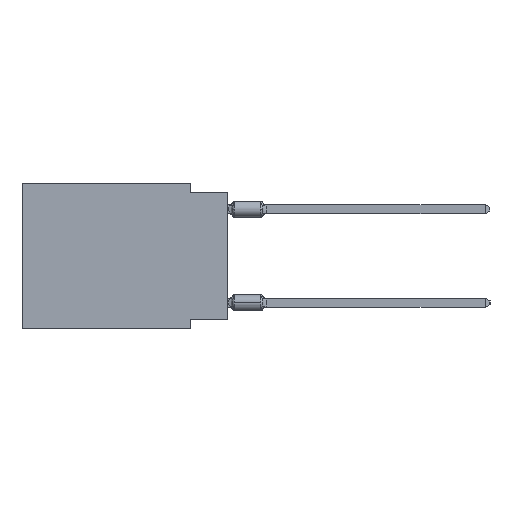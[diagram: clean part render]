
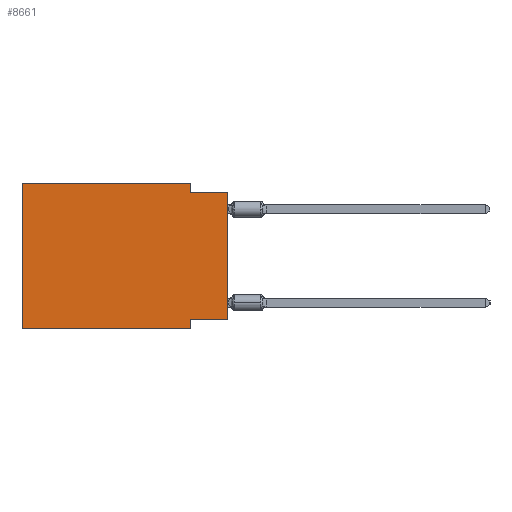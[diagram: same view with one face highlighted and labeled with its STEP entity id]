
A CAD part, left-side view. The second image highlights one B-rep face of the part: STEP entity #8661.
In plain terms, the highlighted planar face has unit normal (-1, 0, 0).
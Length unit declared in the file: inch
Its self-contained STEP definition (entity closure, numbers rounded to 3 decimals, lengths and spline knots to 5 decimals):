
#216 = CARTESIAN_POINT ( 'NONE',  ( 0., 0.1, -0.025 ) ) ;
#1521 = LINE ( 'NONE', #36367, #37844 ) ;
#1956 = ORIENTED_EDGE ( 'NONE', *, *, #28556, .F. ) ;
#2195 = CARTESIAN_POINT ( 'NONE',  ( 0., 0.1, 0. ) ) ;
#2839 = CARTESIAN_POINT ( 'NONE',  ( 0., 0.55, -0.39 ) ) ;
#4814 = LINE ( 'NONE', #23485, #38915 ) ;
#5425 = ORIENTED_EDGE ( 'NONE', *, *, #21490, .F. ) ;
#6575 = EDGE_CURVE ( 'NONE', #15605, #26968, #23163, .T. ) ;
#7314 = VERTEX_POINT ( 'NONE', #25768 ) ;
#8661 = ADVANCED_FACE ( 'NONE', ( #19843 ), #29776, .F. ) ;
#9729 = ORIENTED_EDGE ( 'NONE', *, *, #18205, .F. ) ;
#10688 = DIRECTION ( 'NONE',  ( 1., 0., 0. ) ) ;
#10963 = DIRECTION ( 'NONE',  ( 0., 0., 1. ) ) ;
#11843 = DIRECTION ( 'NONE',  ( 0., -1., 0. ) ) ;
#12040 = CARTESIAN_POINT ( 'NONE',  ( 0., 0.55, 0. ) ) ;
#12055 = CARTESIAN_POINT ( 'NONE',  ( 0., 0.1, -0.39 ) ) ;
#12072 = VERTEX_POINT ( 'NONE', #216 ) ;
#12468 = DIRECTION ( 'NONE',  ( 0., 0., 1. ) ) ;
#13388 = ORIENTED_EDGE ( 'NONE', *, *, #16372, .T. ) ;
#13749 = DIRECTION ( 'NONE',  ( 0., 1., 0. ) ) ;
#14763 = VECTOR ( 'NONE', #12468, 39.37008 ) ;
#15605 = VERTEX_POINT ( 'NONE', #2839 ) ;
#16372 = EDGE_CURVE ( 'NONE', #22951, #7314, #34476, .T. ) ;
#16384 = DIRECTION ( 'NONE',  ( 0., 0., -1. ) ) ;
#17668 = LINE ( 'NONE', #12040, #34386 ) ;
#17761 = DIRECTION ( 'NONE',  ( 0., 0., -1. ) ) ;
#18205 = EDGE_CURVE ( 'NONE', #35127, #26968, #38156, .T. ) ;
#19767 = VECTOR ( 'NONE', #17761, 39.37008 ) ;
#19843 = FACE_OUTER_BOUND ( 'NONE', #28396, .T. ) ;
#19909 = CARTESIAN_POINT ( 'NONE',  ( 0., 0.1, -0.39 ) ) ;
#20731 = ORIENTED_EDGE ( 'NONE', *, *, #25065, .F. ) ;
#21490 = EDGE_CURVE ( 'NONE', #22951, #35127, #4814, .T. ) ;
#21963 = CARTESIAN_POINT ( 'NONE',  ( 0., 0., -0.365 ) ) ;
#22441 = CARTESIAN_POINT ( 'NONE',  ( 0., 0.55, 0. ) ) ;
#22951 = VERTEX_POINT ( 'NONE', #21963 ) ;
#23114 = EDGE_CURVE ( 'NONE', #15605, #38725, #27157, .T. ) ;
#23163 = LINE ( 'NONE', #36211, #34443 ) ;
#23334 = DIRECTION ( 'NONE',  ( 0., 0., -1. ) ) ;
#23485 = CARTESIAN_POINT ( 'NONE',  ( 0., 0., -0.365 ) ) ;
#23658 = VECTOR ( 'NONE', #10963, 39.37008 ) ;
#24679 = CARTESIAN_POINT ( 'NONE',  ( 0., 0.1, 0. ) ) ;
#25065 = EDGE_CURVE ( 'NONE', #38725, #37426, #17668, .T. ) ;
#25768 = CARTESIAN_POINT ( 'NONE',  ( 0., 0., -0.025 ) ) ;
#26687 = LINE ( 'NONE', #2195, #19767 ) ;
#26968 = VERTEX_POINT ( 'NONE', #12055 ) ;
#27035 = DIRECTION ( 'NONE',  ( 0., -1., 0. ) ) ;
#27157 = LINE ( 'NONE', #39802, #23658 ) ;
#28396 = EDGE_LOOP ( 'NONE', ( #13388, #1956, #31101, #20731, #38252, #34993, #9729, #5425 ) ) ;
#28556 = EDGE_CURVE ( 'NONE', #12072, #7314, #1521, .T. ) ;
#29776 = PLANE ( 'NONE',  #38803 ) ;
#30192 = DIRECTION ( 'NONE',  ( 0., -1., 0. ) ) ;
#31101 = ORIENTED_EDGE ( 'NONE', *, *, #39812, .F. ) ;
#32109 = VECTOR ( 'NONE', #16384, 39.37008 ) ;
#32486 = CARTESIAN_POINT ( 'NONE',  ( 0., 0.1, -0.365 ) ) ;
#34272 = CARTESIAN_POINT ( 'NONE',  ( 0., 0., 0. ) ) ;
#34386 = VECTOR ( 'NONE', #11843, 39.37008 ) ;
#34443 = VECTOR ( 'NONE', #30192, 39.37008 ) ;
#34476 = LINE ( 'NONE', #34272, #14763 ) ;
#34993 = ORIENTED_EDGE ( 'NONE', *, *, #6575, .T. ) ;
#35127 = VERTEX_POINT ( 'NONE', #32486 ) ;
#35804 = CARTESIAN_POINT ( 'NONE',  ( 0., 0.55, 0. ) ) ;
#36211 = CARTESIAN_POINT ( 'NONE',  ( 0., 0.55, -0.39 ) ) ;
#36367 = CARTESIAN_POINT ( 'NONE',  ( 0., 0., -0.025 ) ) ;
#37426 = VERTEX_POINT ( 'NONE', #24679 ) ;
#37844 = VECTOR ( 'NONE', #27035, 39.37008 ) ;
#38156 = LINE ( 'NONE', #19909, #32109 ) ;
#38252 = ORIENTED_EDGE ( 'NONE', *, *, #23114, .F. ) ;
#38725 = VERTEX_POINT ( 'NONE', #22441 ) ;
#38803 = AXIS2_PLACEMENT_3D ( 'NONE', #35804, #10688, #23334 ) ;
#38915 = VECTOR ( 'NONE', #13749, 39.37008 ) ;
#39802 = CARTESIAN_POINT ( 'NONE',  ( 0., 0.55, 0. ) ) ;
#39812 = EDGE_CURVE ( 'NONE', #37426, #12072, #26687, .T. ) ;
